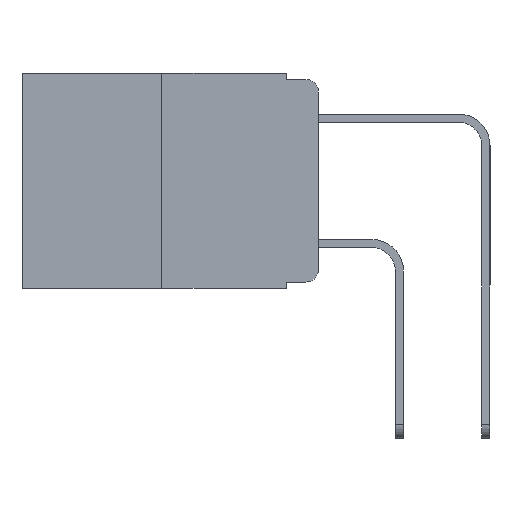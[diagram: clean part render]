
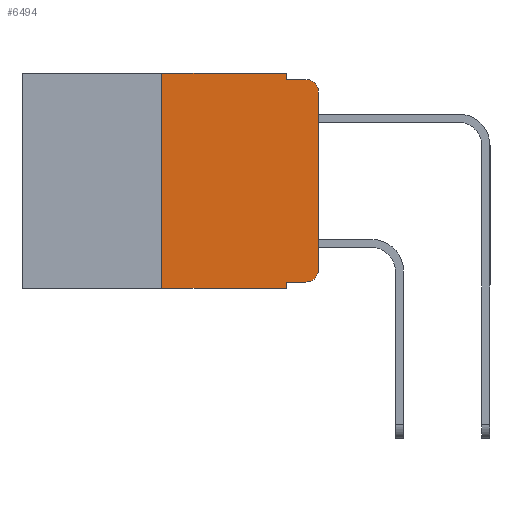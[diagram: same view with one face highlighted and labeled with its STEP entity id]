
A CAD part, left-side view. The second image highlights one B-rep face of the part: STEP entity #6494.
In plain terms, the highlighted planar face has unit normal (-1, 0, 0).
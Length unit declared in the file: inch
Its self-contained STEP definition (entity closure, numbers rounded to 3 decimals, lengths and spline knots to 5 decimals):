
#113 = DIRECTION ( 'NONE',  ( 0., -1., 0. ) ) ;
#142 = VERTEX_POINT ( 'NONE', #9166 ) ;
#643 = FACE_OUTER_BOUND ( 'NONE', #920, .T. ) ;
#920 = EDGE_LOOP ( 'NONE', ( #1468, #6033, #11670, #9498, #4806, #2058, #11501, #7509, #1680, #5178 ) ) ;
#1155 = VECTOR ( 'NONE', #6503, 39.37008 ) ;
#1221 = AXIS2_PLACEMENT_3D ( 'NONE', #12652, #8925, #12199 ) ;
#1468 = ORIENTED_EDGE ( 'NONE', *, *, #4128, .T. ) ;
#1680 = ORIENTED_EDGE ( 'NONE', *, *, #5939, .T. ) ;
#1704 = CARTESIAN_POINT ( 'NONE',  ( 0., 0.051, -0.333 ) ) ;
#1937 = CARTESIAN_POINT ( 'NONE',  ( 0., 0.051, 0. ) ) ;
#2058 = ORIENTED_EDGE ( 'NONE', *, *, #7345, .F. ) ;
#2205 = LINE ( 'NONE', #8108, #10577 ) ;
#2521 = CARTESIAN_POINT ( 'NONE',  ( 0., 0.02, -0.03 ) ) ;
#2773 = VERTEX_POINT ( 'NONE', #12870 ) ;
#3067 = VECTOR ( 'NONE', #5063, 39.37008 ) ;
#3319 = DIRECTION ( 'NONE',  ( 0., -1., 0. ) ) ;
#3390 = CARTESIAN_POINT ( 'NONE',  ( 0., 0.051, -0.01 ) ) ;
#3516 = DIRECTION ( 'NONE',  ( 0., -1., 0. ) ) ;
#3621 = EDGE_CURVE ( 'NONE', #142, #2773, #5533, .T. ) ;
#3636 = CARTESIAN_POINT ( 'NONE',  ( 0., 0.473, 0. ) ) ;
#3675 = AXIS2_PLACEMENT_3D ( 'NONE', #2521, #10172, #3697 ) ;
#3688 = PLANE ( 'NONE',  #13532 ) ;
#3697 = DIRECTION ( 'NONE',  ( 0., 0., -1. ) ) ;
#4128 = EDGE_CURVE ( 'NONE', #2773, #9142, #10451, .T. ) ;
#4697 = CARTESIAN_POINT ( 'NONE',  ( 0., 0.051, -0.01 ) ) ;
#4806 = ORIENTED_EDGE ( 'NONE', *, *, #11603, .F. ) ;
#4873 = DIRECTION ( 'NONE',  ( 0., 0., -1. ) ) ;
#5063 = DIRECTION ( 'NONE',  ( 0., 0., 1. ) ) ;
#5145 = LINE ( 'NONE', #7897, #10775 ) ;
#5178 = ORIENTED_EDGE ( 'NONE', *, *, #3621, .T. ) ;
#5468 = VERTEX_POINT ( 'NONE', #1704 ) ;
#5533 = CIRCLE ( 'NONE', #1221, 0.02 ) ;
#5747 = VERTEX_POINT ( 'NONE', #9885 ) ;
#5939 = EDGE_CURVE ( 'NONE', #5468, #142, #2205, .T. ) ;
#6033 = ORIENTED_EDGE ( 'NONE', *, *, #12365, .T. ) ;
#6333 = VERTEX_POINT ( 'NONE', #3390 ) ;
#6494 = ADVANCED_FACE ( 'NONE', ( #643 ), #3688, .F. ) ;
#6503 = DIRECTION ( 'NONE',  ( 0., 0., -1. ) ) ;
#6650 = EDGE_CURVE ( 'NONE', #5468, #9187, #12962, .T. ) ;
#7345 = EDGE_CURVE ( 'NONE', #11935, #12585, #12124, .T. ) ;
#7382 = CARTESIAN_POINT ( 'NONE',  ( 0., 0.25, 0. ) ) ;
#7509 = ORIENTED_EDGE ( 'NONE', *, *, #6650, .F. ) ;
#7682 = CIRCLE ( 'NONE', #3675, 0.02 ) ;
#7897 = CARTESIAN_POINT ( 'NONE',  ( 0., 0.473, 0. ) ) ;
#7937 = DIRECTION ( 'NONE',  ( 0., -1., 0. ) ) ;
#8108 = CARTESIAN_POINT ( 'NONE',  ( 0., 0.051, -0.333 ) ) ;
#8353 = DIRECTION ( 'NONE',  ( 0., 0., 1. ) ) ;
#8768 = EDGE_CURVE ( 'NONE', #9615, #6333, #12903, .T. ) ;
#8925 = DIRECTION ( 'NONE',  ( -1., 0., 0. ) ) ;
#9142 = VERTEX_POINT ( 'NONE', #10457 ) ;
#9166 = CARTESIAN_POINT ( 'NONE',  ( 0., 0.02, -0.333 ) ) ;
#9187 = VERTEX_POINT ( 'NONE', #9441 ) ;
#9441 = CARTESIAN_POINT ( 'NONE',  ( 0., 0.051, -0.343 ) ) ;
#9498 = ORIENTED_EDGE ( 'NONE', *, *, #8768, .F. ) ;
#9586 = CARTESIAN_POINT ( 'NONE',  ( 0., 0.051, 0. ) ) ;
#9615 = VERTEX_POINT ( 'NONE', #11381 ) ;
#9636 = LINE ( 'NONE', #10904, #12520 ) ;
#9885 = CARTESIAN_POINT ( 'NONE',  ( 0., 0.02, -0.01 ) ) ;
#10083 = VECTOR ( 'NONE', #10618, 39.37008 ) ;
#10114 = VECTOR ( 'NONE', #7937, 39.37008 ) ;
#10172 = DIRECTION ( 'NONE',  ( -1., 0., 0. ) ) ;
#10451 = LINE ( 'NONE', #12630, #13032 ) ;
#10457 = CARTESIAN_POINT ( 'NONE',  ( 0., 0., -0.03 ) ) ;
#10577 = VECTOR ( 'NONE', #113, 39.37008 ) ;
#10618 = DIRECTION ( 'NONE',  ( 0., 0., -1. ) ) ;
#10775 = VECTOR ( 'NONE', #3516, 39.37008 ) ;
#10904 = CARTESIAN_POINT ( 'NONE',  ( 0., 0.473, -0.343 ) ) ;
#11260 = DIRECTION ( 'NONE',  ( 1., 0., 0. ) ) ;
#11381 = CARTESIAN_POINT ( 'NONE',  ( 0., 0.051, 0. ) ) ;
#11501 = ORIENTED_EDGE ( 'NONE', *, *, #13443, .T. ) ;
#11603 = EDGE_CURVE ( 'NONE', #12585, #9615, #5145, .T. ) ;
#11620 = EDGE_CURVE ( 'NONE', #6333, #5747, #13004, .T. ) ;
#11670 = ORIENTED_EDGE ( 'NONE', *, *, #11620, .F. ) ;
#11935 = VERTEX_POINT ( 'NONE', #12761 ) ;
#12124 = LINE ( 'NONE', #12559, #3067 ) ;
#12199 = DIRECTION ( 'NONE',  ( 0., 0., -1. ) ) ;
#12365 = EDGE_CURVE ( 'NONE', #9142, #5747, #7682, .T. ) ;
#12520 = VECTOR ( 'NONE', #3319, 39.37008 ) ;
#12559 = CARTESIAN_POINT ( 'NONE',  ( 0., 0.25, 0. ) ) ;
#12585 = VERTEX_POINT ( 'NONE', #7382 ) ;
#12630 = CARTESIAN_POINT ( 'NONE',  ( 0., 0., 0. ) ) ;
#12652 = CARTESIAN_POINT ( 'NONE',  ( 0., 0.02, -0.313 ) ) ;
#12761 = CARTESIAN_POINT ( 'NONE',  ( 0., 0.25, -0.343 ) ) ;
#12870 = CARTESIAN_POINT ( 'NONE',  ( 0., 0., -0.313 ) ) ;
#12903 = LINE ( 'NONE', #1937, #1155 ) ;
#12962 = LINE ( 'NONE', #9586, #10083 ) ;
#13004 = LINE ( 'NONE', #4697, #10114 ) ;
#13032 = VECTOR ( 'NONE', #8353, 39.37008 ) ;
#13443 = EDGE_CURVE ( 'NONE', #11935, #9187, #9636, .T. ) ;
#13532 = AXIS2_PLACEMENT_3D ( 'NONE', #3636, #11260, #4873 ) ;
